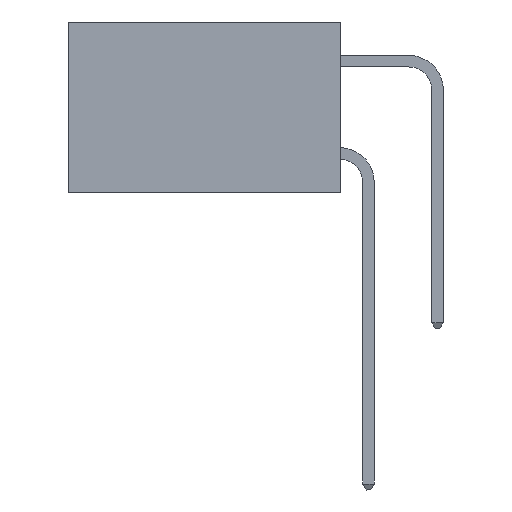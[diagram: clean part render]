
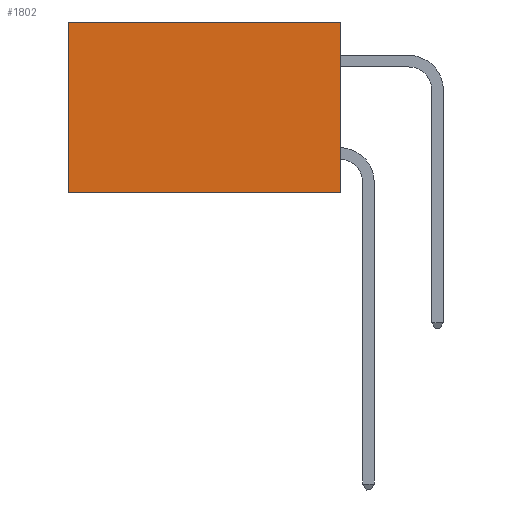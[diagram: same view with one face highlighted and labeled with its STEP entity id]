
A CAD part, left-side view. The second image highlights one B-rep face of the part: STEP entity #1802.
In plain terms, the highlighted planar face has unit normal (-1, 0, 0).
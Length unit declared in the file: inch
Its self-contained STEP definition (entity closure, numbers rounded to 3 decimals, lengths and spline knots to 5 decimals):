
#50 = CARTESIAN_POINT ( 'NONE',  ( 0.277, 0., 0. ) ) ;
#629 = CARTESIAN_POINT ( 'NONE',  ( 0.277, 0.59, -0.37 ) ) ;
#775 = VERTEX_POINT ( 'NONE', #50 ) ;
#857 = DIRECTION ( 'NONE',  ( 0., 1., 0. ) ) ;
#893 = AXIS2_PLACEMENT_3D ( 'NONE', #6236, #8100, #8083 ) ;
#1010 = LINE ( 'NONE', #629, #4911 ) ;
#1036 = ORIENTED_EDGE ( 'NONE', *, *, #9177, .T. ) ;
#1059 = ORIENTED_EDGE ( 'NONE', *, *, #9011, .F. ) ;
#1143 = ORIENTED_EDGE ( 'NONE', *, *, #4108, .F. ) ;
#1186 = EDGE_CURVE ( 'NONE', #775, #7335, #2169, .T. ) ;
#1254 = ORIENTED_EDGE ( 'NONE', *, *, #1186, .T. ) ;
#1492 = DIRECTION ( 'NONE',  ( 0., 0., -1. ) ) ;
#1802 = ADVANCED_FACE ( 'NONE', ( #7613 ), #6019, .F. ) ;
#2166 = CARTESIAN_POINT ( 'NONE',  ( 0.277, 0., -0.37 ) ) ;
#2169 = LINE ( 'NONE', #8480, #8065 ) ;
#2322 = VECTOR ( 'NONE', #5169, 39.37008 ) ;
#2432 = VERTEX_POINT ( 'NONE', #7221 ) ;
#2706 = CARTESIAN_POINT ( 'NONE',  ( 0.277, 0., -0.37 ) ) ;
#3246 = EDGE_LOOP ( 'NONE', ( #1036, #1059, #1143, #1254 ) ) ;
#4108 = EDGE_CURVE ( 'NONE', #775, #8163, #9376, .T. ) ;
#4911 = VECTOR ( 'NONE', #1492, 39.37008 ) ;
#5169 = DIRECTION ( 'NONE',  ( 0., 1., 0. ) ) ;
#5690 = CARTESIAN_POINT ( 'NONE',  ( 0.277, 0., -0.37 ) ) ;
#5816 = DIRECTION ( 'NONE',  ( 0., 0., -1. ) ) ;
#6019 = PLANE ( 'NONE',  #893 ) ;
#6236 = CARTESIAN_POINT ( 'NONE',  ( 0.277, 0., -0.37 ) ) ;
#6303 = LINE ( 'NONE', #2166, #2322 ) ;
#6842 = CARTESIAN_POINT ( 'NONE',  ( 0.277, 0.59, 0. ) ) ;
#7221 = CARTESIAN_POINT ( 'NONE',  ( 0.277, 0.59, -0.37 ) ) ;
#7335 = VERTEX_POINT ( 'NONE', #6842 ) ;
#7613 = FACE_OUTER_BOUND ( 'NONE', #3246, .T. ) ;
#7730 = VECTOR ( 'NONE', #5816, 39.37008 ) ;
#8065 = VECTOR ( 'NONE', #857, 39.37008 ) ;
#8083 = DIRECTION ( 'NONE',  ( 0., 0., -1. ) ) ;
#8100 = DIRECTION ( 'NONE',  ( 1., 0., 0. ) ) ;
#8163 = VERTEX_POINT ( 'NONE', #2706 ) ;
#8480 = CARTESIAN_POINT ( 'NONE',  ( 0.277, 0., 0. ) ) ;
#9011 = EDGE_CURVE ( 'NONE', #8163, #2432, #6303, .T. ) ;
#9177 = EDGE_CURVE ( 'NONE', #7335, #2432, #1010, .T. ) ;
#9376 = LINE ( 'NONE', #5690, #7730 ) ;
